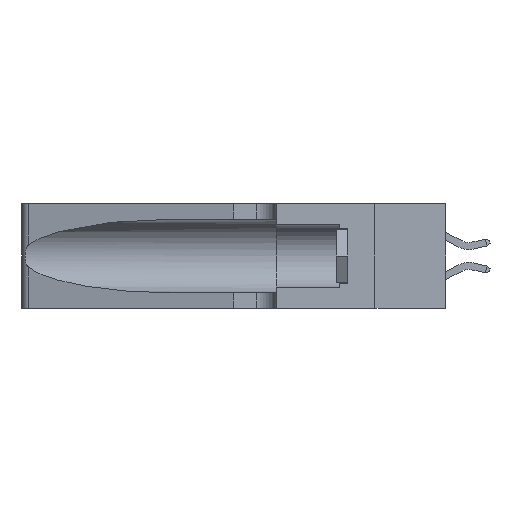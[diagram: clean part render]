
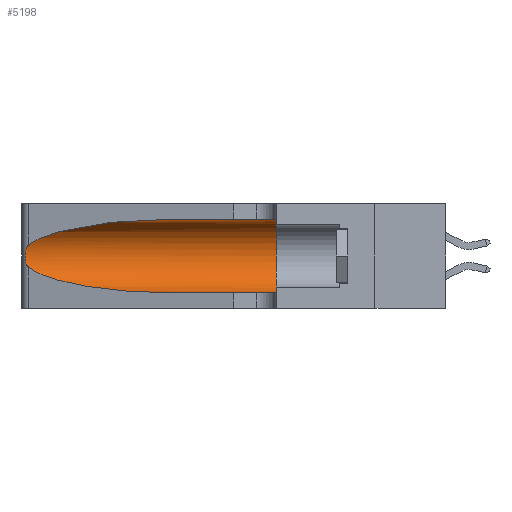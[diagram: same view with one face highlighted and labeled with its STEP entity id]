
A CAD part, left-side view. The second image highlights one B-rep face of the part: STEP entity #5198.
In plain terms, the highlighted cylindrical face has radius 3.308 mm (diameter 6.617 mm), a partial arc.
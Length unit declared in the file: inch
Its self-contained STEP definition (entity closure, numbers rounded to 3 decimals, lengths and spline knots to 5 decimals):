
#313 = CARTESIAN_POINT ( 'NONE',  ( 0.1305, 0.35, 0.185 ) ) ;
#323 = CARTESIAN_POINT ( 'NONE',  ( 0.25555, 1.22994, 0.2215 ) ) ;
#432 = CARTESIAN_POINT ( 'NONE',  ( 0.25555, 1.22993, 0.14849 ) ) ;
#468 = ORIENTED_EDGE ( 'NONE', *, *, #9507, .T. ) ;
#609 = FACE_OUTER_BOUND ( 'NONE', #5418, .T. ) ;
#1164 = ORIENTED_EDGE ( 'NONE', *, *, #23686, .T. ) ;
#1644 = CARTESIAN_POINT ( 'NONE',  ( 0.1305, 1.61858, 0.05475 ) ) ;
#1799 = VERTEX_POINT ( 'NONE', #18847 ) ;
#2752 = EDGE_CURVE ( 'NONE', #13622, #26462, #21796, .T. ) ;
#2923 = DIRECTION ( 'NONE',  ( 0., 0., 1. ) ) ;
#4064 =( BOUNDED_CURVE ( )  B_SPLINE_CURVE ( 3, ( #29762, #20129, #22555, #7880 ),
 .UNSPECIFIED., .F., .F. ) 
 B_SPLINE_CURVE_WITH_KNOTS ( ( 4, 4 ),
 ( 1.5708, 2.84003 ),
 .UNSPECIFIED. ) 
 CURVE ( )  GEOMETRIC_REPRESENTATION_ITEM ( )  RATIONAL_B_SPLINE_CURVE ( ( 1., 0.87, 0.87, 1. ) ) 
 REPRESENTATION_ITEM ( '' )  );
#4256 = DIRECTION ( 'NONE',  ( 0., -1., 0. ) ) ;
#4771 = CARTESIAN_POINT ( 'NONE',  ( 0.1305, 1.61858, 0.31525 ) ) ;
#5198 = ADVANCED_FACE ( 'NONE', ( #609 ), #11834, .F. ) ;
#5418 = EDGE_LOOP ( 'NONE', ( #468, #12913, #31519, #1164, #6523, #25515 ) ) ;
#5530 = CARTESIAN_POINT ( 'NONE',  ( 0.25787, 1.23484, 0.2124 ) ) ;
#6460 = CIRCLE ( 'NONE', #17702, 0.13025 ) ;
#6481 = CARTESIAN_POINT ( 'NONE',  ( 0.18966, 0.96281, 0.05475 ) ) ;
#6523 = ORIENTED_EDGE ( 'NONE', *, *, #25215, .F. ) ;
#7359 = DIRECTION ( 'NONE',  ( 0., -1., 0. ) ) ;
#7633 = CARTESIAN_POINT ( 'NONE',  ( 0.1305, 0.35, 0.05475 ) ) ;
#7880 = CARTESIAN_POINT ( 'NONE',  ( 0.25487, 1.22718, 0.22369 ) ) ;
#8130 = CARTESIAN_POINT ( 'NONE',  ( 0.26018, 1.23835, 0.19895 ) ) ;
#9507 = EDGE_CURVE ( 'NONE', #13622, #14482, #4064, .T. ) ;
#9582 = VECTOR ( 'NONE', #7359, 39.37008 ) ;
#10428 = CARTESIAN_POINT ( 'NONE',  ( 0.1305, 0.72297, 0.31525 ) ) ;
#10679 = CARTESIAN_POINT ( 'NONE',  ( 0.26075, 1.23896, 0.178 ) ) ;
#11443 = DIRECTION ( 'NONE',  ( 0., 0., -1. ) ) ;
#11474 = CARTESIAN_POINT ( 'NONE',  ( 0.25487, 1.22718, 0.22369 ) ) ;
#11498 = CARTESIAN_POINT ( 'NONE',  ( 0.25487, 1.22718, 0.14631 ) ) ;
#11834 = CYLINDRICAL_SURFACE ( 'NONE', #19083, 0.13025 ) ;
#12898 = LINE ( 'NONE', #1644, #19346 ) ;
#12913 = ORIENTED_EDGE ( 'NONE', *, *, #14952, .T. ) ;
#13153 = CARTESIAN_POINT ( 'NONE',  ( 0.25856, 1.23593, 0.16098 ) ) ;
#13622 = VERTEX_POINT ( 'NONE', #10428 ) ;
#14482 = VERTEX_POINT ( 'NONE', #11474 ) ;
#14952 = EDGE_CURVE ( 'NONE', #14482, #1799, #27931, .T. ) ;
#15601 = CARTESIAN_POINT ( 'NONE',  ( 0.25639, 1.23186, 0.15144 ) ) ;
#17702 = AXIS2_PLACEMENT_3D ( 'NONE', #313, #17935, #2923 ) ;
#17935 = DIRECTION ( 'NONE',  ( 0., 1., 0. ) ) ;
#17938 = CARTESIAN_POINT ( 'NONE',  ( 0.25487, 1.22718, 0.22369 ) ) ;
#18043 = CARTESIAN_POINT ( 'NONE',  ( 0.25487, 1.22718, 0.14631 ) ) ;
#18847 = CARTESIAN_POINT ( 'NONE',  ( 0.25487, 1.22718, 0.14631 ) ) ;
#19083 = AXIS2_PLACEMENT_3D ( 'NONE', #21084, #25934, #11443 ) ;
#19346 = VECTOR ( 'NONE', #4256, 39.37008 ) ;
#19476 = CARTESIAN_POINT ( 'NONE',  ( 0.1305, 0.72297, 0.05475 ) ) ;
#20005 =( BOUNDED_CURVE ( )  B_SPLINE_CURVE ( 3, ( #11498, #30919, #6481, #23679 ),
 .UNSPECIFIED., .F., .F. ) 
 B_SPLINE_CURVE_WITH_KNOTS ( ( 4, 4 ),
 ( 3.44316, 4.71239 ),
 .UNSPECIFIED. ) 
 CURVE ( )  GEOMETRIC_REPRESENTATION_ITEM ( )  RATIONAL_B_SPLINE_CURVE ( ( 1., 0.87, 0.87, 1. ) ) 
 REPRESENTATION_ITEM ( '' )  );
#20129 = CARTESIAN_POINT ( 'NONE',  ( 0.18966, 0.96281, 0.31525 ) ) ;
#20355 = CARTESIAN_POINT ( 'NONE',  ( 0.25639, 1.23184, 0.21858 ) ) ;
#21084 = CARTESIAN_POINT ( 'NONE',  ( 0.1305, 1.61858, 0.185 ) ) ;
#21651 = VERTEX_POINT ( 'NONE', #19476 ) ;
#21796 = LINE ( 'NONE', #4771, #9582 ) ;
#22555 = CARTESIAN_POINT ( 'NONE',  ( 0.2373, 1.15595, 0.28018 ) ) ;
#22784 = CARTESIAN_POINT ( 'NONE',  ( 0.25854, 1.2359, 0.20912 ) ) ;
#23679 = CARTESIAN_POINT ( 'NONE',  ( 0.1305, 0.72297, 0.05475 ) ) ;
#23686 = EDGE_CURVE ( 'NONE', #21651, #23884, #12898, .T. ) ;
#23884 = VERTEX_POINT ( 'NONE', #7633 ) ;
#25207 = CARTESIAN_POINT ( 'NONE',  ( 0.26075, 1.23896, 0.19203 ) ) ;
#25215 = EDGE_CURVE ( 'NONE', #26462, #23884, #6460, .T. ) ;
#25515 = ORIENTED_EDGE ( 'NONE', *, *, #2752, .F. ) ;
#25934 = DIRECTION ( 'NONE',  ( 0., -1., 0. ) ) ;
#26462 = VERTEX_POINT ( 'NONE', #27288 ) ;
#27288 = CARTESIAN_POINT ( 'NONE',  ( 0.1305, 0.35, 0.31525 ) ) ;
#27630 = CARTESIAN_POINT ( 'NONE',  ( 0.26017, 1.23833, 0.17102 ) ) ;
#27931 = B_SPLINE_CURVE_WITH_KNOTS ( 'NONE', 3,
 ( #17938, #323, #20355, #5530, #22784, #8130, #25207, #10679, #27630, #13153, #30111, #15601, #432, #18043 ),
 .UNSPECIFIED., .F., .F.,
 ( 4, 2, 2, 2, 2, 2, 4 ),
 ( 0., 0.00027, 0.00053, 0.00107, 0.0016, 0.00187, 0.00214 ),
 .UNSPECIFIED. ) ;
#29762 = CARTESIAN_POINT ( 'NONE',  ( 0.1305, 0.72297, 0.31525 ) ) ;
#30111 = CARTESIAN_POINT ( 'NONE',  ( 0.25789, 1.23486, 0.15765 ) ) ;
#30919 = CARTESIAN_POINT ( 'NONE',  ( 0.2373, 1.15595, 0.08982 ) ) ;
#31519 = ORIENTED_EDGE ( 'NONE', *, *, #31644, .T. ) ;
#31644 = EDGE_CURVE ( 'NONE', #1799, #21651, #20005, .T. ) ;
